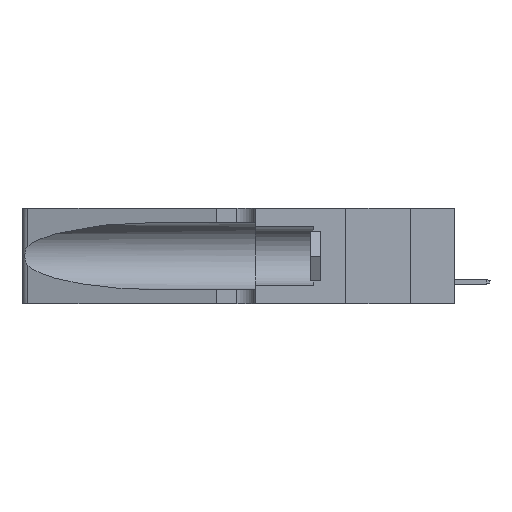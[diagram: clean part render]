
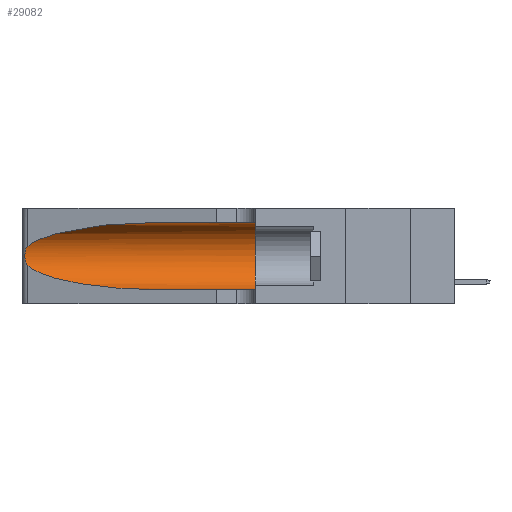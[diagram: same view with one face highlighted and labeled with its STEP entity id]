
A CAD part, left-side view. The second image highlights one B-rep face of the part: STEP entity #29082.
In plain terms, the highlighted cylindrical face has radius 3.308 mm (diameter 6.617 mm), a partial arc.
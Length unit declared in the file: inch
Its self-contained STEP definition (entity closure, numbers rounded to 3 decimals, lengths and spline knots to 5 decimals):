
#1433 = CARTESIAN_POINT ( 'NONE',  ( 0.25789, 1.23486, 0.15765 ) ) ;
#1614 =( BOUNDED_CURVE ( )  B_SPLINE_CURVE ( 3, ( #2290, #17802, #22892, #28138 ),
 .UNSPECIFIED., .F., .T. ) 
 B_SPLINE_CURVE_WITH_KNOTS ( ( 4, 4 ),
 ( 1.5708, 2.84003 ),
 .UNSPECIFIED. ) 
 CURVE ( )  GEOMETRIC_REPRESENTATION_ITEM ( )  RATIONAL_B_SPLINE_CURVE ( ( 1., 0.87, 0.87, 1. ) ) 
 REPRESENTATION_ITEM ( '' )  );
#1930 = CARTESIAN_POINT ( 'NONE',  ( 0.26018, 1.23835, 0.19895 ) ) ;
#1933 = ORIENTED_EDGE ( 'NONE', *, *, #19210, .T. ) ;
#2290 = CARTESIAN_POINT ( 'NONE',  ( 0.1305, 0.72297, 0.31525 ) ) ;
#4467 = CARTESIAN_POINT ( 'NONE',  ( 0.26075, 1.23896, 0.178 ) ) ;
#5068 =( BOUNDED_CURVE ( )  B_SPLINE_CURVE ( 3, ( #31929, #8798, #29414, #26880 ),
 .UNSPECIFIED., .F., .T. ) 
 B_SPLINE_CURVE_WITH_KNOTS ( ( 4, 4 ),
 ( 3.44316, 4.71239 ),
 .UNSPECIFIED. ) 
 CURVE ( )  GEOMETRIC_REPRESENTATION_ITEM ( )  RATIONAL_B_SPLINE_CURVE ( ( 1., 0.87, 0.87, 1. ) ) 
 REPRESENTATION_ITEM ( '' )  );
#5402 = CARTESIAN_POINT ( 'NONE',  ( 0.1305, 1.61858, 0.31525 ) ) ;
#6727 = AXIS2_PLACEMENT_3D ( 'NONE', #28657, #10574, #26447 ) ;
#6786 = CARTESIAN_POINT ( 'NONE',  ( 0.1305, 0.35, 0.05475 ) ) ;
#6827 = CARTESIAN_POINT ( 'NONE',  ( 0.26017, 1.23833, 0.17102 ) ) ;
#6971 = FACE_OUTER_BOUND ( 'NONE', #13848, .T. ) ;
#7287 = VERTEX_POINT ( 'NONE', #10272 ) ;
#8798 = CARTESIAN_POINT ( 'NONE',  ( 0.2373, 1.15595, 0.08982 ) ) ;
#8807 = EDGE_CURVE ( 'NONE', #7287, #25125, #25047, .T. ) ;
#9362 = CARTESIAN_POINT ( 'NONE',  ( 0.25639, 1.23186, 0.15144 ) ) ;
#9491 = VERTEX_POINT ( 'NONE', #23839 ) ;
#9522 = CARTESIAN_POINT ( 'NONE',  ( 0.25856, 1.23593, 0.16098 ) ) ;
#10272 = CARTESIAN_POINT ( 'NONE',  ( 0.25487, 1.22718, 0.22369 ) ) ;
#10574 = DIRECTION ( 'NONE',  ( 0., 1., 0. ) ) ;
#11393 = ORIENTED_EDGE ( 'NONE', *, *, #26085, .F. ) ;
#11536 = VERTEX_POINT ( 'NONE', #23575 ) ;
#13848 = EDGE_LOOP ( 'NONE', ( #1933, #23852, #25919, #19675, #11393, #25726 ) ) ;
#14573 = CARTESIAN_POINT ( 'NONE',  ( 0.1305, 1.61858, 0.185 ) ) ;
#17100 = DIRECTION ( 'NONE',  ( 0., -1., 0. ) ) ;
#17258 = DIRECTION ( 'NONE',  ( 0., 0., -1. ) ) ;
#17635 = AXIS2_PLACEMENT_3D ( 'NONE', #14573, #17100, #17258 ) ;
#17802 = CARTESIAN_POINT ( 'NONE',  ( 0.18966, 0.96281, 0.31525 ) ) ;
#18224 = LINE ( 'NONE', #5402, #27472 ) ;
#19210 = EDGE_CURVE ( 'NONE', #9491, #7287, #1614, .T. ) ;
#19328 = CARTESIAN_POINT ( 'NONE',  ( 0.25555, 1.22993, 0.14849 ) ) ;
#19667 = CARTESIAN_POINT ( 'NONE',  ( 0.25487, 1.22718, 0.14631 ) ) ;
#19675 = ORIENTED_EDGE ( 'NONE', *, *, #24709, .T. ) ;
#21975 = VECTOR ( 'NONE', #28314, 39.37008 ) ;
#22133 = EDGE_CURVE ( 'NONE', #25125, #25810, #5068, .T. ) ;
#22362 = CIRCLE ( 'NONE', #6727, 0.13025 ) ;
#22526 = CYLINDRICAL_SURFACE ( 'NONE', #17635, 0.13025 ) ;
#22543 = CARTESIAN_POINT ( 'NONE',  ( 0.25787, 1.23484, 0.2124 ) ) ;
#22892 = CARTESIAN_POINT ( 'NONE',  ( 0.2373, 1.15595, 0.28018 ) ) ;
#23575 = CARTESIAN_POINT ( 'NONE',  ( 0.1305, 0.35, 0.31525 ) ) ;
#23839 = CARTESIAN_POINT ( 'NONE',  ( 0.1305, 0.72297, 0.31525 ) ) ;
#23852 = ORIENTED_EDGE ( 'NONE', *, *, #8807, .T. ) ;
#24577 = CARTESIAN_POINT ( 'NONE',  ( 0.26075, 1.23896, 0.19203 ) ) ;
#24709 = EDGE_CURVE ( 'NONE', #25810, #26704, #25606, .T. ) ;
#24742 = CARTESIAN_POINT ( 'NONE',  ( 0.25854, 1.2359, 0.20912 ) ) ;
#25047 = B_SPLINE_CURVE_WITH_KNOTS ( 'NONE', 3,
 ( #29813, #25074, #30311, #22543, #24742, #1930, #24577, #4467, #6827, #9522, #1433, #9362, #19328, #19667 ),
 .UNSPECIFIED., .F., .F.,
 ( 4, 2, 2, 2, 2, 2, 4 ),
 ( 0., 0.00027, 0.00053, 0.00107, 0.0016, 0.00187, 0.00214 ),
 .UNSPECIFIED. ) ;
#25074 = CARTESIAN_POINT ( 'NONE',  ( 0.25555, 1.22994, 0.2215 ) ) ;
#25125 = VERTEX_POINT ( 'NONE', #33325 ) ;
#25606 = LINE ( 'NONE', #30842, #21975 ) ;
#25726 = ORIENTED_EDGE ( 'NONE', *, *, #32812, .F. ) ;
#25810 = VERTEX_POINT ( 'NONE', #29524 ) ;
#25919 = ORIENTED_EDGE ( 'NONE', *, *, #22133, .T. ) ;
#26085 = EDGE_CURVE ( 'NONE', #11536, #26704, #22362, .T. ) ;
#26447 = DIRECTION ( 'NONE',  ( 0., 0., 1. ) ) ;
#26704 = VERTEX_POINT ( 'NONE', #6786 ) ;
#26880 = CARTESIAN_POINT ( 'NONE',  ( 0.1305, 0.72297, 0.05475 ) ) ;
#27472 = VECTOR ( 'NONE', #31696, 39.37008 ) ;
#28138 = CARTESIAN_POINT ( 'NONE',  ( 0.25487, 1.22718, 0.22369 ) ) ;
#28314 = DIRECTION ( 'NONE',  ( 0., -1., 0. ) ) ;
#28657 = CARTESIAN_POINT ( 'NONE',  ( 0.1305, 0.35, 0.185 ) ) ;
#29082 = ADVANCED_FACE ( 'NONE', ( #6971 ), #22526, .F. ) ;
#29414 = CARTESIAN_POINT ( 'NONE',  ( 0.18966, 0.96281, 0.05475 ) ) ;
#29524 = CARTESIAN_POINT ( 'NONE',  ( 0.1305, 0.72297, 0.05475 ) ) ;
#29813 = CARTESIAN_POINT ( 'NONE',  ( 0.25487, 1.22718, 0.22369 ) ) ;
#30311 = CARTESIAN_POINT ( 'NONE',  ( 0.25639, 1.23184, 0.21858 ) ) ;
#30842 = CARTESIAN_POINT ( 'NONE',  ( 0.1305, 1.61858, 0.05475 ) ) ;
#31696 = DIRECTION ( 'NONE',  ( 0., -1., 0. ) ) ;
#31929 = CARTESIAN_POINT ( 'NONE',  ( 0.25487, 1.22718, 0.14631 ) ) ;
#32812 = EDGE_CURVE ( 'NONE', #9491, #11536, #18224, .T. ) ;
#33325 = CARTESIAN_POINT ( 'NONE',  ( 0.25487, 1.22718, 0.14631 ) ) ;
